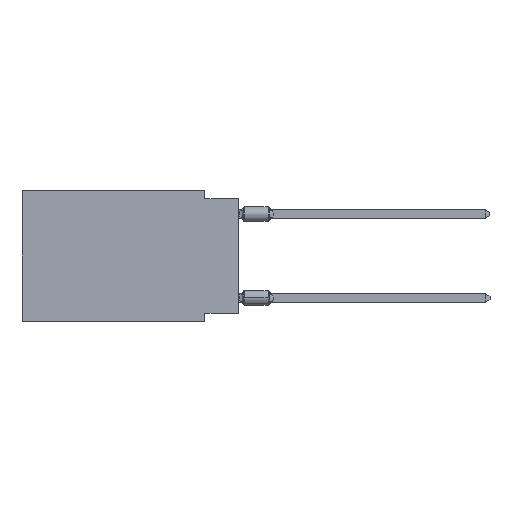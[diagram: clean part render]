
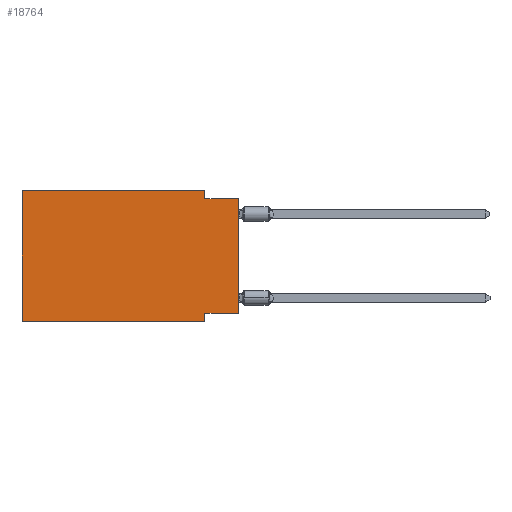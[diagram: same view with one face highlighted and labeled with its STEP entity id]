
A CAD part, left-side view. The second image highlights one B-rep face of the part: STEP entity #18764.
In plain terms, the highlighted planar face has unit normal (-1, 0, 0).
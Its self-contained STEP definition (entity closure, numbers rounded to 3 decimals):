
#384 = EDGE_CURVE ( 'NONE', #2217, #4612, #2568, .T. ) ;
#621 = ORIENTED_EDGE ( 'NONE', *, *, #16242, .T. ) ;
#988 = VERTEX_POINT ( 'NONE', #12493 ) ;
#1155 = CARTESIAN_POINT ( 'NONE',  ( 0., 2.54, -0.635 ) ) ;
#1381 = VECTOR ( 'NONE', #5545, 1000. ) ;
#1664 = EDGE_LOOP ( 'NONE', ( #621, #18965, #14600, #2232, #7229, #7820, #19504, #20570 ) ) ;
#2104 = VERTEX_POINT ( 'NONE', #7966 ) ;
#2217 = VERTEX_POINT ( 'NONE', #12703 ) ;
#2232 = ORIENTED_EDGE ( 'NONE', *, *, #3556, .F. ) ;
#2568 = LINE ( 'NONE', #11990, #7339 ) ;
#2784 = DIRECTION ( 'NONE',  ( 1., 0., 0. ) ) ;
#3139 = DIRECTION ( 'NONE',  ( 0., 0., -1. ) ) ;
#3387 = LINE ( 'NONE', #18071, #13424 ) ;
#3556 = EDGE_CURVE ( 'NONE', #4612, #12614, #13403, .T. ) ;
#3772 = EDGE_CURVE ( 'NONE', #10909, #2104, #8662, .T. ) ;
#4612 = VERTEX_POINT ( 'NONE', #14316 ) ;
#4873 = LINE ( 'NONE', #14720, #16250 ) ;
#4926 = EDGE_CURVE ( 'NONE', #988, #10923, #18703, .T. ) ;
#5029 = EDGE_CURVE ( 'NONE', #10923, #14442, #4873, .T. ) ;
#5192 = DIRECTION ( 'NONE',  ( 0., -1., 0. ) ) ;
#5302 = DIRECTION ( 'NONE',  ( 0., -1., 0. ) ) ;
#5545 = DIRECTION ( 'NONE',  ( 0., 1., 0. ) ) ;
#7143 = DIRECTION ( 'NONE',  ( 0., 0., 1. ) ) ;
#7229 = ORIENTED_EDGE ( 'NONE', *, *, #384, .F. ) ;
#7339 = VECTOR ( 'NONE', #7143, 1000. ) ;
#7678 = CARTESIAN_POINT ( 'NONE',  ( 0., 16.383, 0. ) ) ;
#7820 = ORIENTED_EDGE ( 'NONE', *, *, #16559, .T. ) ;
#7966 = CARTESIAN_POINT ( 'NONE',  ( 0., 0., -0.635 ) ) ;
#8662 = LINE ( 'NONE', #8773, #16042 ) ;
#8773 = CARTESIAN_POINT ( 'NONE',  ( 0., 0., -0.635 ) ) ;
#8942 = DIRECTION ( 'NONE',  ( 0., 0., 1. ) ) ;
#9321 = VECTOR ( 'NONE', #8942, 1000. ) ;
#10909 = VERTEX_POINT ( 'NONE', #1155 ) ;
#10923 = VERTEX_POINT ( 'NONE', #14379 ) ;
#11990 = CARTESIAN_POINT ( 'NONE',  ( 0., 16.383, 0. ) ) ;
#12419 = FACE_OUTER_BOUND ( 'NONE', #1664, .T. ) ;
#12493 = CARTESIAN_POINT ( 'NONE',  ( 0., 0., -9.271 ) ) ;
#12614 = VERTEX_POINT ( 'NONE', #16942 ) ;
#12703 = CARTESIAN_POINT ( 'NONE',  ( 0., 16.383, -9.906 ) ) ;
#13122 = CARTESIAN_POINT ( 'NONE',  ( 0., 16.383, -9.906 ) ) ;
#13403 = LINE ( 'NONE', #18149, #14304 ) ;
#13424 = VECTOR ( 'NONE', #17964, 1000. ) ;
#14115 = LINE ( 'NONE', #20668, #9321 ) ;
#14304 = VECTOR ( 'NONE', #5192, 1000. ) ;
#14316 = CARTESIAN_POINT ( 'NONE',  ( 0., 16.383, 0. ) ) ;
#14379 = CARTESIAN_POINT ( 'NONE',  ( 0., 2.54, -9.271 ) ) ;
#14442 = VERTEX_POINT ( 'NONE', #19472 ) ;
#14600 = ORIENTED_EDGE ( 'NONE', *, *, #15337, .F. ) ;
#14720 = CARTESIAN_POINT ( 'NONE',  ( 0., 2.54, -9.906 ) ) ;
#15337 = EDGE_CURVE ( 'NONE', #12614, #10909, #3387, .T. ) ;
#16042 = VECTOR ( 'NONE', #5302, 1000. ) ;
#16242 = EDGE_CURVE ( 'NONE', #988, #2104, #14115, .T. ) ;
#16250 = VECTOR ( 'NONE', #3139, 1000. ) ;
#16559 = EDGE_CURVE ( 'NONE', #2217, #14442, #17972, .T. ) ;
#16942 = CARTESIAN_POINT ( 'NONE',  ( 0., 2.54, 0. ) ) ;
#17374 = DIRECTION ( 'NONE',  ( 0., 0., -1. ) ) ;
#17964 = DIRECTION ( 'NONE',  ( 0., 0., -1. ) ) ;
#17972 = LINE ( 'NONE', #13122, #21020 ) ;
#17995 = AXIS2_PLACEMENT_3D ( 'NONE', #7678, #2784, #17374 ) ;
#18071 = CARTESIAN_POINT ( 'NONE',  ( 0., 2.54, 0. ) ) ;
#18149 = CARTESIAN_POINT ( 'NONE',  ( 0., 16.383, 0. ) ) ;
#18703 = LINE ( 'NONE', #19020, #1381 ) ;
#18764 = ADVANCED_FACE ( 'NONE', ( #12419 ), #20919, .F. ) ;
#18965 = ORIENTED_EDGE ( 'NONE', *, *, #3772, .F. ) ;
#19020 = CARTESIAN_POINT ( 'NONE',  ( 0., 0., -9.271 ) ) ;
#19472 = CARTESIAN_POINT ( 'NONE',  ( 0., 2.54, -9.906 ) ) ;
#19504 = ORIENTED_EDGE ( 'NONE', *, *, #5029, .F. ) ;
#19686 = DIRECTION ( 'NONE',  ( 0., -1., 0. ) ) ;
#20570 = ORIENTED_EDGE ( 'NONE', *, *, #4926, .F. ) ;
#20668 = CARTESIAN_POINT ( 'NONE',  ( 0., 0., 0. ) ) ;
#20919 = PLANE ( 'NONE',  #17995 ) ;
#21020 = VECTOR ( 'NONE', #19686, 1000. ) ;
